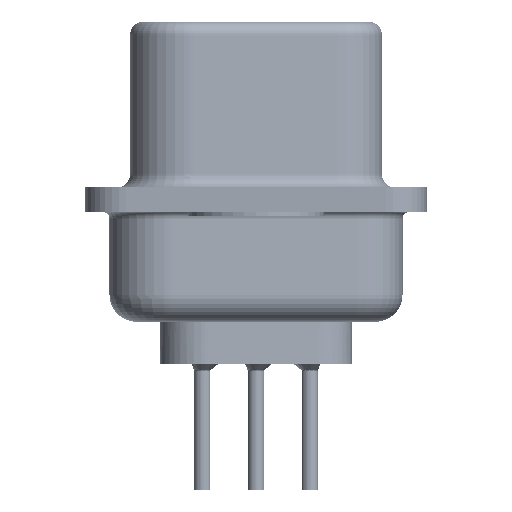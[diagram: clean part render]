
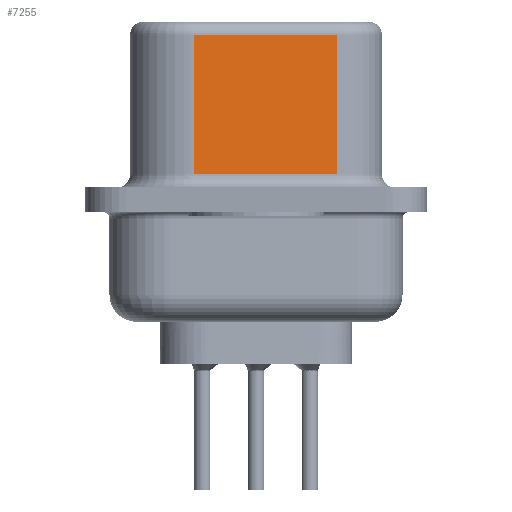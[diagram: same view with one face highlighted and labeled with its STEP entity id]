
A CAD part, left-side view. The second image highlights one B-rep face of the part: STEP entity #7255.
In plain terms, the highlighted planar face has unit normal (-0.985, -0.174, 0).
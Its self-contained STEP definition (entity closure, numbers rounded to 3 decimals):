
#658 = VERTEX_POINT ( 'NONE', #34719 ) ;
#1913 = EDGE_LOOP ( 'NONE', ( #8889, #26504, #29255, #25663 ) ) ;
#3811 = CARTESIAN_POINT ( 'NONE',  ( 3.62, 2.293, 6.07 ) ) ;
#3983 = EDGE_CURVE ( 'NONE', #16822, #22719, #20133, .T. ) ;
#5382 = CARTESIAN_POINT ( 'NONE',  ( 4.551, -2.987, 6.07 ) ) ;
#7255 = ADVANCED_FACE ( 'NONE', ( #17253 ), #14404, .F. ) ;
#8594 = CARTESIAN_POINT ( 'NONE',  ( 4.551, -2.987, 6.07 ) ) ;
#8649 = AXIS2_PLACEMENT_3D ( 'NONE', #29033, #26018, #20318 ) ;
#8889 = ORIENTED_EDGE ( 'NONE', *, *, #3983, .F. ) ;
#9132 = EDGE_CURVE ( 'NONE', #16822, #13804, #22688, .T. ) ;
#9343 = LINE ( 'NONE', #18093, #34805 ) ;
#13804 = VERTEX_POINT ( 'NONE', #3811 ) ;
#13931 = DIRECTION ( 'NONE',  ( -0.174, 0.985, 0. ) ) ;
#14404 = PLANE ( 'NONE',  #8649 ) ;
#16822 = VERTEX_POINT ( 'NONE', #8594 ) ;
#16920 = EDGE_CURVE ( 'NONE', #658, #22719, #25892, .T. ) ;
#17129 = CARTESIAN_POINT ( 'NONE',  ( 4.551, -2.987, 0.95 ) ) ;
#17253 = FACE_OUTER_BOUND ( 'NONE', #1913, .T. ) ;
#18093 = CARTESIAN_POINT ( 'NONE',  ( 3.62, 2.293, 6.57 ) ) ;
#20133 = LINE ( 'NONE', #31708, #32396 ) ;
#20318 = DIRECTION ( 'NONE',  ( -0.174, 0.985, 0. ) ) ;
#22688 = LINE ( 'NONE', #5382, #22707 ) ;
#22707 = VECTOR ( 'NONE', #13931, 1000. ) ;
#22719 = VERTEX_POINT ( 'NONE', #36286 ) ;
#23371 = DIRECTION ( 'NONE',  ( 0., 0., -1. ) ) ;
#24185 = DIRECTION ( 'NONE',  ( 0., 0., -1. ) ) ;
#25663 = ORIENTED_EDGE ( 'NONE', *, *, #16920, .T. ) ;
#25892 = LINE ( 'NONE', #17129, #33293 ) ;
#26018 = DIRECTION ( 'NONE',  ( 0.985, 0.174, 0. ) ) ;
#26504 = ORIENTED_EDGE ( 'NONE', *, *, #9132, .T. ) ;
#27067 = EDGE_CURVE ( 'NONE', #13804, #658, #9343, .T. ) ;
#28726 = DIRECTION ( 'NONE',  ( 0.174, -0.985, 0. ) ) ;
#29033 = CARTESIAN_POINT ( 'NONE',  ( 4.551, -2.987, 6.57 ) ) ;
#29255 = ORIENTED_EDGE ( 'NONE', *, *, #27067, .T. ) ;
#31708 = CARTESIAN_POINT ( 'NONE',  ( 4.551, -2.987, 6.57 ) ) ;
#32396 = VECTOR ( 'NONE', #23371, 1000. ) ;
#33293 = VECTOR ( 'NONE', #28726, 1000. ) ;
#34719 = CARTESIAN_POINT ( 'NONE',  ( 3.62, 2.293, 0.95 ) ) ;
#34805 = VECTOR ( 'NONE', #24185, 1000. ) ;
#36286 = CARTESIAN_POINT ( 'NONE',  ( 4.551, -2.987, 0.95 ) ) ;
